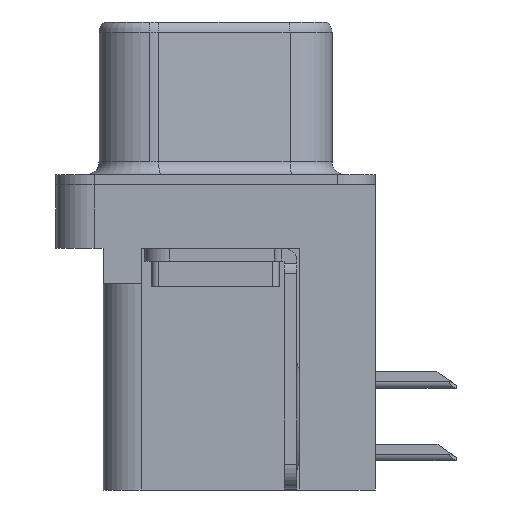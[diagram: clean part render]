
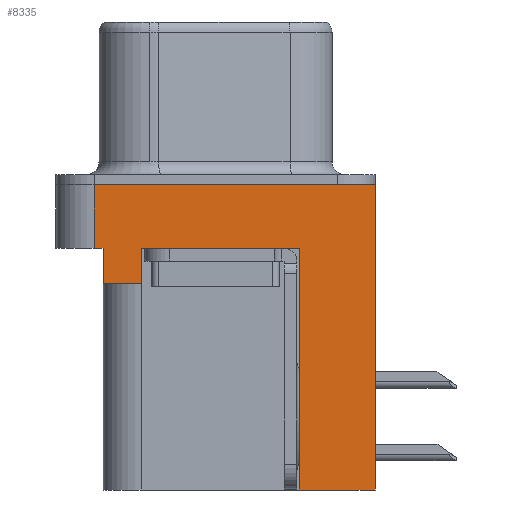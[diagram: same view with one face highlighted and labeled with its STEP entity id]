
A CAD part, left-side view. The second image highlights one B-rep face of the part: STEP entity #8335.
In plain terms, the highlighted planar face has unit normal (-1, 0, 0).
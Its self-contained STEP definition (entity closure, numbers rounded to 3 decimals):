
#188 = DIRECTION ( 'NONE',  ( 0., 1., 0. ) ) ;
#212 = CARTESIAN_POINT ( 'NONE',  ( -2.935, 2.895, -2.5 ) ) ;
#214 = DIRECTION ( 'NONE',  ( 0., -1., 0. ) ) ;
#252 = CARTESIAN_POINT ( 'NONE',  ( -2.935, 4.775, -2.5 ) ) ;
#360 = EDGE_CURVE ( 'NONE', #17254, #14364, #1549, .T. ) ;
#1251 = DIRECTION ( 'NONE',  ( 0., 0., 1. ) ) ;
#1366 = EDGE_CURVE ( 'NONE', #7256, #16540, #7325, .T. ) ;
#1549 = LINE ( 'NONE', #11681, #4218 ) ;
#1598 = DIRECTION ( 'NONE',  ( 0., 1., 0. ) ) ;
#1622 = CARTESIAN_POINT ( 'NONE',  ( -2.935, 4.775, 0. ) ) ;
#1748 = DIRECTION ( 'NONE',  ( 0., 0., 1. ) ) ;
#1815 = CARTESIAN_POINT ( 'NONE',  ( -2.935, -3.295, -12. ) ) ;
#1989 = ORIENTED_EDGE ( 'NONE', *, *, #5523, .F. ) ;
#2224 = LINE ( 'NONE', #8018, #17227 ) ;
#2710 = DIRECTION ( 'NONE',  ( 0., 0., 1. ) ) ;
#3103 = CARTESIAN_POINT ( 'NONE',  ( -2.935, -6.275, -2.5 ) ) ;
#3278 = VECTOR ( 'NONE', #188, 1000. ) ;
#3289 = CARTESIAN_POINT ( 'NONE',  ( -2.935, -6.275, 0. ) ) ;
#3411 = VECTOR ( 'NONE', #14993, 1000. ) ;
#4068 = LINE ( 'NONE', #3289, #3411 ) ;
#4072 = VECTOR ( 'NONE', #1598, 1000. ) ;
#4084 = CARTESIAN_POINT ( 'NONE',  ( -2.935, 4.425, -3.9 ) ) ;
#4218 = VECTOR ( 'NONE', #1748, 1000. ) ;
#4571 = CARTESIAN_POINT ( 'NONE',  ( -2.935, 4.775, -2.5 ) ) ;
#4576 = DIRECTION ( 'NONE',  ( 0., 0., 1. ) ) ;
#4782 = DIRECTION ( 'NONE',  ( -1., 0., 0. ) ) ;
#4868 = CARTESIAN_POINT ( 'NONE',  ( -2.935, -3.295, -2.5 ) ) ;
#4983 = VERTEX_POINT ( 'NONE', #4571 ) ;
#5482 = VECTOR ( 'NONE', #214, 1000. ) ;
#5523 = EDGE_CURVE ( 'NONE', #17216, #7389, #4068, .T. ) ;
#5899 = CARTESIAN_POINT ( 'NONE',  ( -2.935, -6.275, 0. ) ) ;
#6083 = DIRECTION ( 'NONE',  ( 0., 0., 1. ) ) ;
#6221 = ORIENTED_EDGE ( 'NONE', *, *, #1366, .F. ) ;
#7256 = VERTEX_POINT ( 'NONE', #9747 ) ;
#7325 = LINE ( 'NONE', #4084, #9786 ) ;
#7389 = VERTEX_POINT ( 'NONE', #5899 ) ;
#7494 = LINE ( 'NONE', #12679, #5482 ) ;
#7700 = LINE ( 'NONE', #252, #8840 ) ;
#7723 = EDGE_CURVE ( 'NONE', #16436, #17254, #17752, .T. ) ;
#8018 = CARTESIAN_POINT ( 'NONE',  ( -2.935, -6.275, -2.5 ) ) ;
#8216 = VECTOR ( 'NONE', #1251, 1000. ) ;
#8335 = ADVANCED_FACE ( 'NONE', ( #10102 ), #17670, .T. ) ;
#8474 = CARTESIAN_POINT ( 'NONE',  ( -2.935, -3.295, -12. ) ) ;
#8479 = AXIS2_PLACEMENT_3D ( 'NONE', #10296, #4782, #6083 ) ;
#8732 = CARTESIAN_POINT ( 'NONE',  ( -2.935, 4.425, -3.9 ) ) ;
#8840 = VECTOR ( 'NONE', #4576, 1000. ) ;
#9747 = CARTESIAN_POINT ( 'NONE',  ( -2.935, 4.425, -3.9 ) ) ;
#9786 = VECTOR ( 'NONE', #2710, 1000. ) ;
#9939 = CARTESIAN_POINT ( 'NONE',  ( -2.935, 2.895, -3.9 ) ) ;
#10009 = ORIENTED_EDGE ( 'NONE', *, *, #18380, .T. ) ;
#10102 = FACE_OUTER_BOUND ( 'NONE', #15903, .T. ) ;
#10296 = CARTESIAN_POINT ( 'NONE',  ( -2.935, -6.275, -2.5 ) ) ;
#10785 = EDGE_CURVE ( 'NONE', #4983, #16540, #2224, .T. ) ;
#11472 = CARTESIAN_POINT ( 'NONE',  ( -2.935, 4.425, -2.5 ) ) ;
#11570 = ORIENTED_EDGE ( 'NONE', *, *, #7723, .F. ) ;
#11681 = CARTESIAN_POINT ( 'NONE',  ( -2.935, -3.295, -12. ) ) ;
#11921 = CARTESIAN_POINT ( 'NONE',  ( -2.935, 2.895, -3.9 ) ) ;
#12679 = CARTESIAN_POINT ( 'NONE',  ( -2.935, -6.275, -2.5 ) ) ;
#12750 = EDGE_CURVE ( 'NONE', #16613, #7256, #18256, .T. ) ;
#12781 = DIRECTION ( 'NONE',  ( 0., 0., 1. ) ) ;
#12787 = ORIENTED_EDGE ( 'NONE', *, *, #12750, .F. ) ;
#13135 = VERTEX_POINT ( 'NONE', #212 ) ;
#13410 = ORIENTED_EDGE ( 'NONE', *, *, #18122, .T. ) ;
#13664 = EDGE_CURVE ( 'NONE', #4983, #17216, #7700, .T. ) ;
#13941 = ORIENTED_EDGE ( 'NONE', *, *, #360, .F. ) ;
#14109 = ORIENTED_EDGE ( 'NONE', *, *, #13664, .F. ) ;
#14364 = VERTEX_POINT ( 'NONE', #4868 ) ;
#14712 = CARTESIAN_POINT ( 'NONE',  ( -2.935, -6.275, -12. ) ) ;
#14713 = VECTOR ( 'NONE', #12781, 1000. ) ;
#14857 = ORIENTED_EDGE ( 'NONE', *, *, #10785, .T. ) ;
#14993 = DIRECTION ( 'NONE',  ( 0., -1., 0. ) ) ;
#15843 = LINE ( 'NONE', #9939, #8216 ) ;
#15903 = EDGE_LOOP ( 'NONE', ( #1989, #14109, #14857, #6221, #12787, #16706, #10009, #13941, #11570, #13410 ) ) ;
#16436 = VERTEX_POINT ( 'NONE', #14712 ) ;
#16540 = VERTEX_POINT ( 'NONE', #11472 ) ;
#16613 = VERTEX_POINT ( 'NONE', #11921 ) ;
#16706 = ORIENTED_EDGE ( 'NONE', *, *, #17564, .T. ) ;
#16755 = DIRECTION ( 'NONE',  ( 0., -1., 0. ) ) ;
#17216 = VERTEX_POINT ( 'NONE', #1622 ) ;
#17227 = VECTOR ( 'NONE', #16755, 1000. ) ;
#17254 = VERTEX_POINT ( 'NONE', #1815 ) ;
#17564 = EDGE_CURVE ( 'NONE', #16613, #13135, #15843, .T. ) ;
#17605 = LINE ( 'NONE', #3103, #14713 ) ;
#17670 = PLANE ( 'NONE',  #8479 ) ;
#17752 = LINE ( 'NONE', #8474, #4072 ) ;
#18122 = EDGE_CURVE ( 'NONE', #16436, #7389, #17605, .T. ) ;
#18256 = LINE ( 'NONE', #8732, #3278 ) ;
#18380 = EDGE_CURVE ( 'NONE', #13135, #14364, #7494, .T. ) ;
